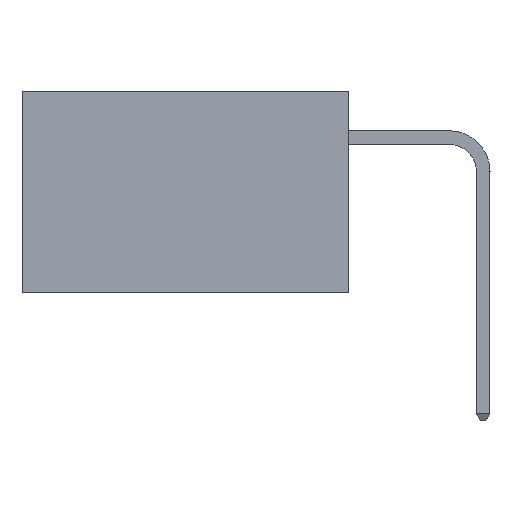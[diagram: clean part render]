
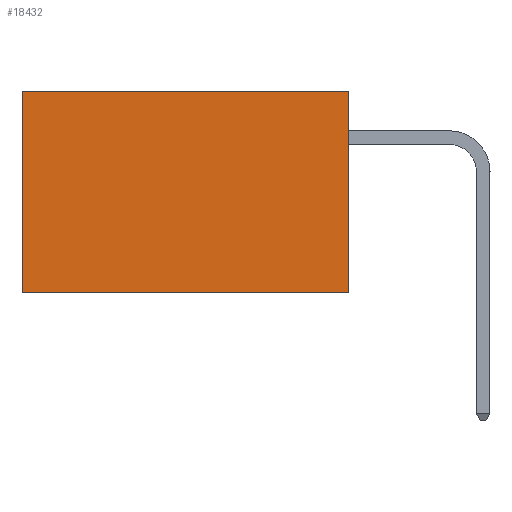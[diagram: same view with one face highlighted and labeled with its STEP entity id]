
A CAD part, left-side view. The second image highlights one B-rep face of the part: STEP entity #18432.
In plain terms, the highlighted planar face has unit normal (-1, 0, 0).
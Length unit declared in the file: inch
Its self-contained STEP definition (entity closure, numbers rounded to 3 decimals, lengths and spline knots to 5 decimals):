
#177 = CARTESIAN_POINT ( 'NONE',  ( 0.2875, 0.6, 0. ) ) ;
#178 = LINE ( 'NONE', #15994, #11607 ) ;
#684 = VECTOR ( 'NONE', #11672, 39.37008 ) ;
#2757 = EDGE_CURVE ( 'NONE', #8185, #7010, #178, .T. ) ;
#5657 = PLANE ( 'NONE',  #14891 ) ;
#6065 = LINE ( 'NONE', #14906, #7511 ) ;
#6276 = DIRECTION ( 'NONE',  ( 0., 1., 0. ) ) ;
#7010 = VERTEX_POINT ( 'NONE', #177 ) ;
#7225 = DIRECTION ( 'NONE',  ( 0., 0., -1. ) ) ;
#7511 = VECTOR ( 'NONE', #6276, 39.37008 ) ;
#7871 = ORIENTED_EDGE ( 'NONE', *, *, #8707, .F. ) ;
#8185 = VERTEX_POINT ( 'NONE', #19036 ) ;
#8707 = EDGE_CURVE ( 'NONE', #15805, #18743, #6065, .T. ) ;
#8905 = CARTESIAN_POINT ( 'NONE',  ( 0.2875, 0., 0. ) ) ;
#8983 = ORIENTED_EDGE ( 'NONE', *, *, #17241, .F. ) ;
#9969 = CARTESIAN_POINT ( 'NONE',  ( 0.2875, 0., 0. ) ) ;
#9978 = VECTOR ( 'NONE', #17501, 39.37008 ) ;
#10200 = CARTESIAN_POINT ( 'NONE',  ( 0.2875, 0.6, 0. ) ) ;
#11607 = VECTOR ( 'NONE', #12695, 39.37008 ) ;
#11672 = DIRECTION ( 'NONE',  ( 0., 0., -1. ) ) ;
#11997 = FACE_OUTER_BOUND ( 'NONE', #15772, .T. ) ;
#12537 = LINE ( 'NONE', #10200, #684 ) ;
#12695 = DIRECTION ( 'NONE',  ( 0., 1., 0. ) ) ;
#13841 = LINE ( 'NONE', #8905, #9978 ) ;
#14891 = AXIS2_PLACEMENT_3D ( 'NONE', #9969, #15744, #7225 ) ;
#14906 = CARTESIAN_POINT ( 'NONE',  ( 0.2875, 0., -0.37 ) ) ;
#15744 = DIRECTION ( 'NONE',  ( 1., 0., 0. ) ) ;
#15761 = EDGE_CURVE ( 'NONE', #7010, #18743, #12537, .T. ) ;
#15772 = EDGE_LOOP ( 'NONE', ( #16912, #7871, #8983, #16072 ) ) ;
#15805 = VERTEX_POINT ( 'NONE', #17525 ) ;
#15994 = CARTESIAN_POINT ( 'NONE',  ( 0.2875, 0., 0. ) ) ;
#16072 = ORIENTED_EDGE ( 'NONE', *, *, #2757, .T. ) ;
#16501 = CARTESIAN_POINT ( 'NONE',  ( 0.2875, 0.6, -0.37 ) ) ;
#16912 = ORIENTED_EDGE ( 'NONE', *, *, #15761, .T. ) ;
#17241 = EDGE_CURVE ( 'NONE', #8185, #15805, #13841, .T. ) ;
#17501 = DIRECTION ( 'NONE',  ( 0., 0., -1. ) ) ;
#17525 = CARTESIAN_POINT ( 'NONE',  ( 0.2875, 0., -0.37 ) ) ;
#18432 = ADVANCED_FACE ( 'NONE', ( #11997 ), #5657, .F. ) ;
#18743 = VERTEX_POINT ( 'NONE', #16501 ) ;
#19036 = CARTESIAN_POINT ( 'NONE',  ( 0.2875, 0., 0. ) ) ;
